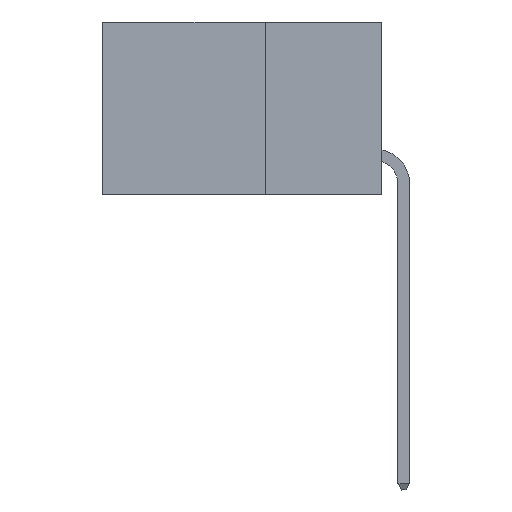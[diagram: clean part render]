
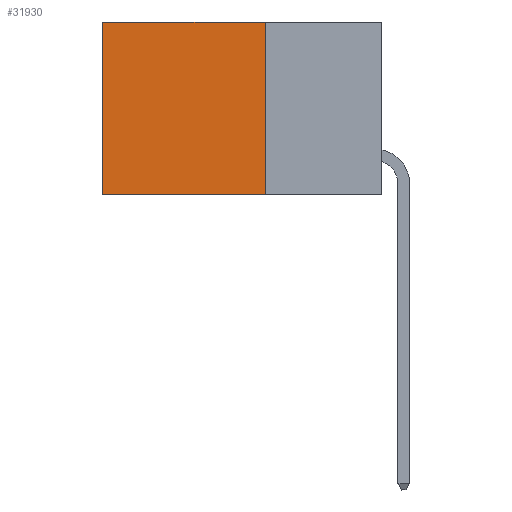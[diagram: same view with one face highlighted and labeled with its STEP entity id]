
A CAD part, left-side view. The second image highlights one B-rep face of the part: STEP entity #31930.
In plain terms, the highlighted planar face has unit normal (-1, 0, 0).
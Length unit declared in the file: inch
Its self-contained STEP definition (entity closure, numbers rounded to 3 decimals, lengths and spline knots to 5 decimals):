
#2589 = LINE ( 'NONE', #19875, #33984 ) ;
#3533 = LINE ( 'NONE', #8029, #10001 ) ;
#3955 = AXIS2_PLACEMENT_3D ( 'NONE', #42560, #20304, #19813 ) ;
#5088 = CARTESIAN_POINT ( 'NONE',  ( 0.2875, 0.25, 0. ) ) ;
#6051 = DIRECTION ( 'NONE',  ( 0., 0., -1. ) ) ;
#8029 = CARTESIAN_POINT ( 'NONE',  ( 0.2875, 0.25, 0. ) ) ;
#8723 = DIRECTION ( 'NONE',  ( 0., 1., 0. ) ) ;
#9334 = EDGE_CURVE ( 'NONE', #33905, #30721, #3533, .T. ) ;
#10001 = VECTOR ( 'NONE', #11645, 39.37008 ) ;
#11645 = DIRECTION ( 'NONE',  ( 0., 0., -1. ) ) ;
#13956 = CARTESIAN_POINT ( 'NONE',  ( 0.2875, 0.6, 0. ) ) ;
#14237 = VECTOR ( 'NONE', #8723, 39.37008 ) ;
#17298 = EDGE_CURVE ( 'NONE', #33905, #25866, #19484, .T. ) ;
#19484 = LINE ( 'NONE', #5088, #14237 ) ;
#19813 = DIRECTION ( 'NONE',  ( 0., 0., -1. ) ) ;
#19875 = CARTESIAN_POINT ( 'NONE',  ( 0.2875, 0.25, -0.37 ) ) ;
#20304 = DIRECTION ( 'NONE',  ( 1., 0., 0. ) ) ;
#23364 = DIRECTION ( 'NONE',  ( 0., 1., 0. ) ) ;
#23401 = CARTESIAN_POINT ( 'NONE',  ( 0.2875, 0.6, 0. ) ) ;
#25866 = VERTEX_POINT ( 'NONE', #23401 ) ;
#27164 = CARTESIAN_POINT ( 'NONE',  ( 0.2875, 0.25, 0. ) ) ;
#27647 = PLANE ( 'NONE',  #3955 ) ;
#27867 = VECTOR ( 'NONE', #6051, 39.37008 ) ;
#28712 = ORIENTED_EDGE ( 'NONE', *, *, #9334, .F. ) ;
#30721 = VERTEX_POINT ( 'NONE', #39854 ) ;
#30878 = FACE_OUTER_BOUND ( 'NONE', #45616, .T. ) ;
#31262 = EDGE_CURVE ( 'NONE', #30721, #43560, #2589, .T. ) ;
#31554 = ORIENTED_EDGE ( 'NONE', *, *, #17298, .T. ) ;
#31930 = ADVANCED_FACE ( 'NONE', ( #30878 ), #27647, .F. ) ;
#31994 = CARTESIAN_POINT ( 'NONE',  ( 0.2875, 0.6, -0.37 ) ) ;
#33820 = LINE ( 'NONE', #13956, #27867 ) ;
#33905 = VERTEX_POINT ( 'NONE', #27164 ) ;
#33984 = VECTOR ( 'NONE', #23364, 39.37008 ) ;
#34626 = ORIENTED_EDGE ( 'NONE', *, *, #31262, .F. ) ;
#37909 = EDGE_CURVE ( 'NONE', #25866, #43560, #33820, .T. ) ;
#39647 = ORIENTED_EDGE ( 'NONE', *, *, #37909, .T. ) ;
#39854 = CARTESIAN_POINT ( 'NONE',  ( 0.2875, 0.25, -0.37 ) ) ;
#42560 = CARTESIAN_POINT ( 'NONE',  ( 0.2875, 0.25, 0. ) ) ;
#43560 = VERTEX_POINT ( 'NONE', #31994 ) ;
#45616 = EDGE_LOOP ( 'NONE', ( #39647, #34626, #28712, #31554 ) ) ;
